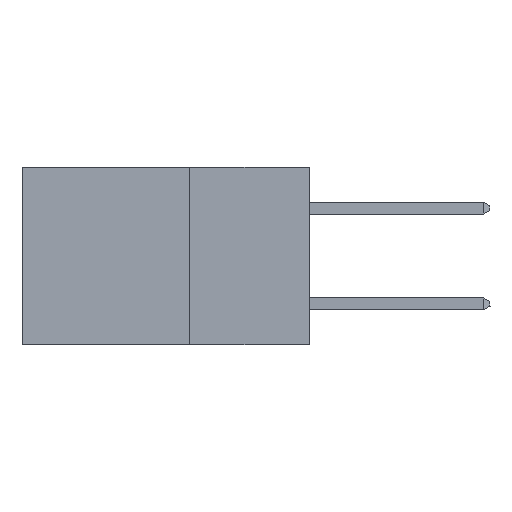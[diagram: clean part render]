
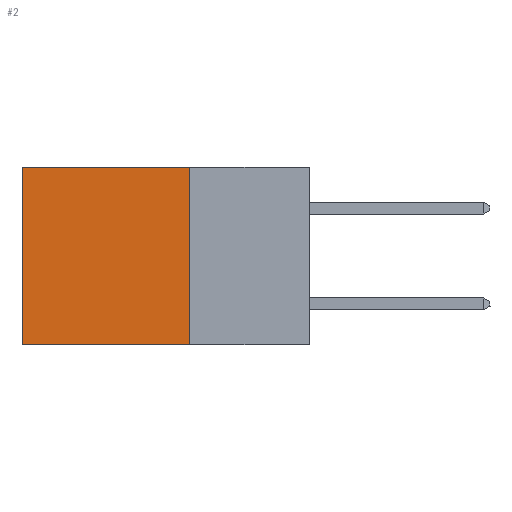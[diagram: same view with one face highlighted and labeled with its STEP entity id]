
A CAD part, left-side view. The second image highlights one B-rep face of the part: STEP entity #2.
In plain terms, the highlighted planar face has unit normal (-1, 0, 0).
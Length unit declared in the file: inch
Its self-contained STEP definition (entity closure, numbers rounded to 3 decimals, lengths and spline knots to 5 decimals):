
#2 = ADVANCED_FACE ( 'NONE', ( #3515 ), #23541, .F. ) ;
#1868 = DIRECTION ( 'NONE',  ( 0., 0., -1. ) ) ;
#3515 = FACE_OUTER_BOUND ( 'NONE', #12872, .T. ) ;
#4737 = LINE ( 'NONE', #20258, #20223 ) ;
#4814 = CARTESIAN_POINT ( 'NONE',  ( 0.2875, 0.25, -0.37 ) ) ;
#5437 = DIRECTION ( 'NONE',  ( 1., 0., 0. ) ) ;
#6053 = EDGE_CURVE ( 'NONE', #14280, #16823, #11248, .T. ) ;
#6284 = DIRECTION ( 'NONE',  ( 0., 0., -1. ) ) ;
#7334 = AXIS2_PLACEMENT_3D ( 'NONE', #22319, #5437, #27741 ) ;
#9266 = CARTESIAN_POINT ( 'NONE',  ( 0.2875, 0.25, 0. ) ) ;
#9304 = CARTESIAN_POINT ( 'NONE',  ( 0.2875, 0.25, 0. ) ) ;
#10546 = ORIENTED_EDGE ( 'NONE', *, *, #24338, .F. ) ;
#10803 = LINE ( 'NONE', #9266, #14803 ) ;
#11248 = LINE ( 'NONE', #22968, #18246 ) ;
#12872 = EDGE_LOOP ( 'NONE', ( #20744, #10546, #28603, #29400 ) ) ;
#14280 = VERTEX_POINT ( 'NONE', #20008 ) ;
#14803 = VECTOR ( 'NONE', #19003, 39.37008 ) ;
#15136 = EDGE_CURVE ( 'NONE', #25214, #26389, #4737, .T. ) ;
#15550 = LINE ( 'NONE', #4814, #21115 ) ;
#16608 = DIRECTION ( 'NONE',  ( 0., 1., 0. ) ) ;
#16823 = VERTEX_POINT ( 'NONE', #21534 ) ;
#18233 = CARTESIAN_POINT ( 'NONE',  ( 0.2875, 0.25, -0.37 ) ) ;
#18246 = VECTOR ( 'NONE', #1868, 39.37008 ) ;
#19003 = DIRECTION ( 'NONE',  ( 0., 1., 0. ) ) ;
#20008 = CARTESIAN_POINT ( 'NONE',  ( 0.2875, 0.6, 0. ) ) ;
#20223 = VECTOR ( 'NONE', #6284, 39.37008 ) ;
#20258 = CARTESIAN_POINT ( 'NONE',  ( 0.2875, 0.25, 0. ) ) ;
#20744 = ORIENTED_EDGE ( 'NONE', *, *, #6053, .T. ) ;
#21115 = VECTOR ( 'NONE', #16608, 39.37008 ) ;
#21534 = CARTESIAN_POINT ( 'NONE',  ( 0.2875, 0.6, -0.37 ) ) ;
#22319 = CARTESIAN_POINT ( 'NONE',  ( 0.2875, 0.25, 0. ) ) ;
#22968 = CARTESIAN_POINT ( 'NONE',  ( 0.2875, 0.6, 0. ) ) ;
#23541 = PLANE ( 'NONE',  #7334 ) ;
#24328 = EDGE_CURVE ( 'NONE', #25214, #14280, #10803, .T. ) ;
#24338 = EDGE_CURVE ( 'NONE', #26389, #16823, #15550, .T. ) ;
#25214 = VERTEX_POINT ( 'NONE', #9304 ) ;
#26389 = VERTEX_POINT ( 'NONE', #18233 ) ;
#27741 = DIRECTION ( 'NONE',  ( 0., 0., -1. ) ) ;
#28603 = ORIENTED_EDGE ( 'NONE', *, *, #15136, .F. ) ;
#29400 = ORIENTED_EDGE ( 'NONE', *, *, #24328, .T. ) ;
